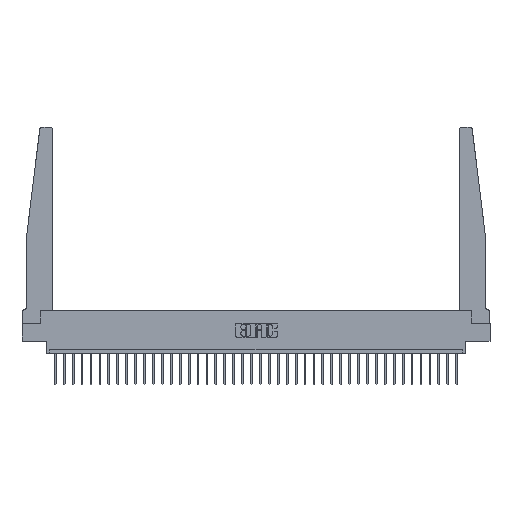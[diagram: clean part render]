
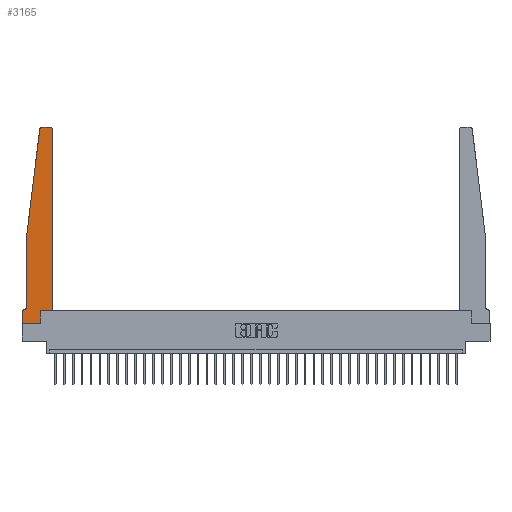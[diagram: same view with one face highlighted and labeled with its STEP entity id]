
A CAD part, top view. The second image highlights one B-rep face of the part: STEP entity #3165.
In plain terms, the highlighted planar face has unit normal (0, 0, 1).
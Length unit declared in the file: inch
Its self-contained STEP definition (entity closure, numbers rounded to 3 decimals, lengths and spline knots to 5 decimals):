
#14 = VECTOR ( 'NONE', #29681, 39.37008 ) ;
#102 = ORIENTED_EDGE ( 'NONE', *, *, #10727, .T. ) ;
#1484 = AXIS2_PLACEMENT_3D ( 'NONE', #14760, #17126, #25043 ) ;
#1715 = CARTESIAN_POINT ( 'NONE',  ( 0., 0., 0.37 ) ) ;
#2579 = DIRECTION ( 'NONE',  ( 0., 1., 0. ) ) ;
#2732 = VECTOR ( 'NONE', #20710, 39.37008 ) ;
#2947 = CARTESIAN_POINT ( 'NONE',  ( 0.2605, 0., 0.37 ) ) ;
#3088 = VECTOR ( 'NONE', #18824, 39.37008 ) ;
#3165 = ADVANCED_FACE ( 'NONE', ( #30394 ), #24835, .T. ) ;
#3741 = VERTEX_POINT ( 'NONE', #2947 ) ;
#4434 = CARTESIAN_POINT ( 'NONE',  ( 0.065, 0.2375, 0.37 ) ) ;
#4618 = CARTESIAN_POINT ( 'NONE',  ( 0., 0.1875, 0.37 ) ) ;
#4914 = VECTOR ( 'NONE', #2579, 39.37008 ) ;
#5552 = EDGE_CURVE ( 'NONE', #13458, #19332, #9478, .T. ) ;
#5604 = LINE ( 'NONE', #10493, #27837 ) ;
#5845 = CARTESIAN_POINT ( 'NONE',  ( 0., 0., 0.37 ) ) ;
#6364 = CIRCLE ( 'NONE', #28996, 0.03 ) ;
#6544 = ORIENTED_EDGE ( 'NONE', *, *, #5552, .T. ) ;
#6844 = CARTESIAN_POINT ( 'NONE',  ( 0.27653, 2.72, 0.37 ) ) ;
#7099 = VERTEX_POINT ( 'NONE', #11607 ) ;
#7155 = LINE ( 'NONE', #14918, #4914 ) ;
#7726 = ORIENTED_EDGE ( 'NONE', *, *, #11802, .T. ) ;
#7855 = CARTESIAN_POINT ( 'NONE',  ( 0.425, 0.18, 0.37 ) ) ;
#7963 = ORIENTED_EDGE ( 'NONE', *, *, #23171, .T. ) ;
#8044 = CARTESIAN_POINT ( 'NONE',  ( 0.425, 2.72, 0.37 ) ) ;
#8183 = ORIENTED_EDGE ( 'NONE', *, *, #28489, .T. ) ;
#8221 = ORIENTED_EDGE ( 'NONE', *, *, #12031, .T. ) ;
#8246 = DIRECTION ( 'NONE',  ( 0., 0., 1. ) ) ;
#9275 = EDGE_CURVE ( 'NONE', #14362, #17934, #19957, .T. ) ;
#9478 = LINE ( 'NONE', #1715, #30643 ) ;
#9877 = DIRECTION ( 'NONE',  ( 0., 0., 1. ) ) ;
#10077 = ORIENTED_EDGE ( 'NONE', *, *, #17826, .T. ) ;
#10490 = VERTEX_POINT ( 'NONE', #25354 ) ;
#10493 = CARTESIAN_POINT ( 'NONE',  ( 0.25, 2.75, 0.37 ) ) ;
#10553 = VERTEX_POINT ( 'NONE', #27904 ) ;
#10727 = EDGE_CURVE ( 'NONE', #28118, #7099, #5604, .T. ) ;
#11058 = CARTESIAN_POINT ( 'NONE',  ( 0.395, 2.75, 0.37 ) ) ;
#11230 = CARTESIAN_POINT ( 'NONE',  ( 0.065, 1.25, 0.37 ) ) ;
#11607 = CARTESIAN_POINT ( 'NONE',  ( 0.27653, 2.75, 0.37 ) ) ;
#11680 = DIRECTION ( 'NONE',  ( 1., 0., 0. ) ) ;
#11802 = EDGE_CURVE ( 'NONE', #10553, #14362, #33345, .T. ) ;
#12031 = EDGE_CURVE ( 'NONE', #20923, #21717, #24032, .T. ) ;
#12353 = DIRECTION ( 'NONE',  ( 0., -1., 0. ) ) ;
#13458 = VERTEX_POINT ( 'NONE', #4618 ) ;
#14330 = EDGE_CURVE ( 'NONE', #21717, #20133, #24216, .T. ) ;
#14362 = VERTEX_POINT ( 'NONE', #26245 ) ;
#14498 = EDGE_CURVE ( 'NONE', #20133, #10490, #16038, .T. ) ;
#14603 = ORIENTED_EDGE ( 'NONE', *, *, #14330, .T. ) ;
#14760 = CARTESIAN_POINT ( 'NONE',  ( 0.015, 0.2375, 0.37 ) ) ;
#14918 = CARTESIAN_POINT ( 'NONE',  ( 0.2605, 0.18, 0.37 ) ) ;
#15646 = CARTESIAN_POINT ( 'NONE',  ( 0., 0., 0.37 ) ) ;
#16009 = CARTESIAN_POINT ( 'NONE',  ( 0.395, 2.72, 0.37 ) ) ;
#16038 = CIRCLE ( 'NONE', #1484, 0.05 ) ;
#17126 = DIRECTION ( 'NONE',  ( 0., 0., -1. ) ) ;
#17145 = DIRECTION ( 'NONE',  ( 1., 0., 0. ) ) ;
#17420 = DIRECTION ( 'NONE',  ( 0., 0., 1. ) ) ;
#17475 = EDGE_CURVE ( 'NONE', #10490, #13458, #19221, .T. ) ;
#17826 = EDGE_CURVE ( 'NONE', #19332, #3741, #21202, .T. ) ;
#17934 = VERTEX_POINT ( 'NONE', #8044 ) ;
#18164 = VECTOR ( 'NONE', #27790, 39.37008 ) ;
#18196 = EDGE_CURVE ( 'NONE', #7099, #20923, #22150, .T. ) ;
#18576 = VECTOR ( 'NONE', #19614, 39.37008 ) ;
#18665 = DIRECTION ( 'NONE',  ( 0., -1., 0. ) ) ;
#18824 = DIRECTION ( 'NONE',  ( -0.122, -0.992, 0. ) ) ;
#18856 = ORIENTED_EDGE ( 'NONE', *, *, #17475, .T. ) ;
#19221 = LINE ( 'NONE', #22243, #14 ) ;
#19332 = VERTEX_POINT ( 'NONE', #5845 ) ;
#19614 = DIRECTION ( 'NONE',  ( 0., 1., 0. ) ) ;
#19957 = LINE ( 'NONE', #32777, #18576 ) ;
#20133 = VERTEX_POINT ( 'NONE', #4434 ) ;
#20668 = ORIENTED_EDGE ( 'NONE', *, *, #14498, .T. ) ;
#20710 = DIRECTION ( 'NONE',  ( 1., 0., 0. ) ) ;
#20923 = VERTEX_POINT ( 'NONE', #27952 ) ;
#21202 = LINE ( 'NONE', #15646, #2732 ) ;
#21343 = CARTESIAN_POINT ( 'NONE',  ( 0.065, 1.25, 0.37 ) ) ;
#21717 = VERTEX_POINT ( 'NONE', #30554 ) ;
#22150 = CIRCLE ( 'NONE', #24830, 0.03 ) ;
#22243 = CARTESIAN_POINT ( 'NONE',  ( 0.065, 0.1875, 0.37 ) ) ;
#22536 = ORIENTED_EDGE ( 'NONE', *, *, #18196, .T. ) ;
#23171 = EDGE_CURVE ( 'NONE', #17934, #28118, #6364, .T. ) ;
#24032 = LINE ( 'NONE', #21343, #3088 ) ;
#24216 = LINE ( 'NONE', #11230, #25206 ) ;
#24830 = AXIS2_PLACEMENT_3D ( 'NONE', #6844, #9877, #17145 ) ;
#24835 = PLANE ( 'NONE',  #30973 ) ;
#25043 = DIRECTION ( 'NONE',  ( -1., 0., 0. ) ) ;
#25206 = VECTOR ( 'NONE', #18665, 39.37008 ) ;
#25354 = CARTESIAN_POINT ( 'NONE',  ( 0.015, 0.1875, 0.37 ) ) ;
#26245 = CARTESIAN_POINT ( 'NONE',  ( 0.425, 0.18, 0.37 ) ) ;
#27755 = EDGE_LOOP ( 'NONE', ( #102, #22536, #8221, #14603, #20668, #18856, #6544, #10077, #8183, #7726, #28467, #7963 ) ) ;
#27790 = DIRECTION ( 'NONE',  ( 1., 0., 0. ) ) ;
#27837 = VECTOR ( 'NONE', #28231, 39.37008 ) ;
#27904 = CARTESIAN_POINT ( 'NONE',  ( 0.2605, 0.18, 0.37 ) ) ;
#27952 = CARTESIAN_POINT ( 'NONE',  ( 0.24675, 2.72367, 0.37 ) ) ;
#28118 = VERTEX_POINT ( 'NONE', #11058 ) ;
#28231 = DIRECTION ( 'NONE',  ( -1., 0., 0. ) ) ;
#28467 = ORIENTED_EDGE ( 'NONE', *, *, #9275, .T. ) ;
#28489 = EDGE_CURVE ( 'NONE', #3741, #10553, #7155, .T. ) ;
#28996 = AXIS2_PLACEMENT_3D ( 'NONE', #16009, #8246, #29342 ) ;
#29342 = DIRECTION ( 'NONE',  ( 1., 0., 0. ) ) ;
#29681 = DIRECTION ( 'NONE',  ( -1., 0., 0. ) ) ;
#29733 = CARTESIAN_POINT ( 'NONE',  ( 0., 0.1875, 0.37 ) ) ;
#30394 = FACE_OUTER_BOUND ( 'NONE', #27755, .T. ) ;
#30554 = CARTESIAN_POINT ( 'NONE',  ( 0.065, 1.25, 0.37 ) ) ;
#30643 = VECTOR ( 'NONE', #12353, 39.37008 ) ;
#30973 = AXIS2_PLACEMENT_3D ( 'NONE', #29733, #17420, #11680 ) ;
#32777 = CARTESIAN_POINT ( 'NONE',  ( 0.425, 0.18, 0.37 ) ) ;
#33345 = LINE ( 'NONE', #7855, #18164 ) ;
